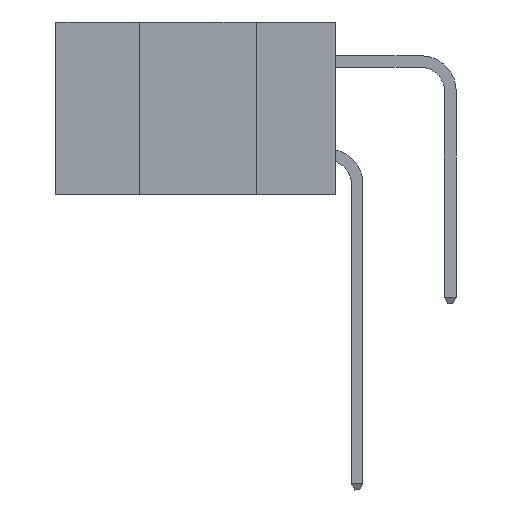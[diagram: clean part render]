
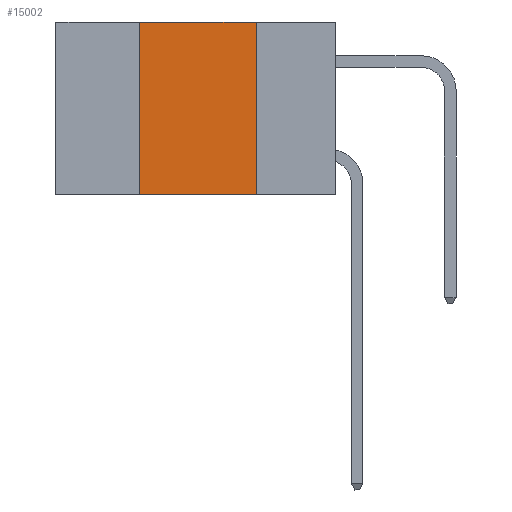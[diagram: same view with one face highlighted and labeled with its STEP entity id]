
A CAD part, left-side view. The second image highlights one B-rep face of the part: STEP entity #15002.
In plain terms, the highlighted planar face has unit normal (-1, 0, 0).
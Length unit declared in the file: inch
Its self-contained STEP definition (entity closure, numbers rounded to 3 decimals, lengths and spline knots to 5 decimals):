
#491 = CARTESIAN_POINT ( 'NONE',  ( 0., 0.17, 0. ) ) ;
#809 = LINE ( 'NONE', #27666, #2516 ) ;
#2391 = ORIENTED_EDGE ( 'NONE', *, *, #9211, .F. ) ;
#2492 = AXIS2_PLACEMENT_3D ( 'NONE', #27152, #17846, #4765 ) ;
#2516 = VECTOR ( 'NONE', #16342, 39.37008 ) ;
#4765 = DIRECTION ( 'NONE',  ( 0., 0., -1. ) ) ;
#4841 = DIRECTION ( 'NONE',  ( 0., 0., 1. ) ) ;
#5401 = LINE ( 'NONE', #14250, #13706 ) ;
#5570 = VERTEX_POINT ( 'NONE', #27965 ) ;
#7860 = CARTESIAN_POINT ( 'NONE',  ( 0., 0.17, 0. ) ) ;
#8285 = DIRECTION ( 'NONE',  ( 0., 0., -1. ) ) ;
#9211 = EDGE_CURVE ( 'NONE', #12813, #18475, #12354, .T. ) ;
#9977 = EDGE_CURVE ( 'NONE', #17232, #18475, #809, .T. ) ;
#11449 = ORIENTED_EDGE ( 'NONE', *, *, #23088, .F. ) ;
#12354 = LINE ( 'NONE', #7860, #24867 ) ;
#12586 = EDGE_LOOP ( 'NONE', ( #2391, #12917, #11449, #15328 ) ) ;
#12813 = VERTEX_POINT ( 'NONE', #491 ) ;
#12845 = CARTESIAN_POINT ( 'NONE',  ( 0., 0.6, 0. ) ) ;
#12917 = ORIENTED_EDGE ( 'NONE', *, *, #27678, .F. ) ;
#13706 = VECTOR ( 'NONE', #4841, 39.37008 ) ;
#14250 = CARTESIAN_POINT ( 'NONE',  ( 0., 0.42, 0. ) ) ;
#14514 = CARTESIAN_POINT ( 'NONE',  ( 0., 0.17, -0.37 ) ) ;
#14952 = VECTOR ( 'NONE', #22011, 39.37008 ) ;
#15002 = ADVANCED_FACE ( 'NONE', ( #15665 ), #22932, .F. ) ;
#15328 = ORIENTED_EDGE ( 'NONE', *, *, #9977, .T. ) ;
#15665 = FACE_OUTER_BOUND ( 'NONE', #12586, .T. ) ;
#16342 = DIRECTION ( 'NONE',  ( 0., -1., 0. ) ) ;
#17232 = VERTEX_POINT ( 'NONE', #17411 ) ;
#17411 = CARTESIAN_POINT ( 'NONE',  ( 0., 0.42, -0.37 ) ) ;
#17846 = DIRECTION ( 'NONE',  ( 1., 0., 0. ) ) ;
#18475 = VERTEX_POINT ( 'NONE', #14514 ) ;
#22011 = DIRECTION ( 'NONE',  ( 0., -1., 0. ) ) ;
#22932 = PLANE ( 'NONE',  #2492 ) ;
#23088 = EDGE_CURVE ( 'NONE', #17232, #5570, #5401, .T. ) ;
#24867 = VECTOR ( 'NONE', #8285, 39.37008 ) ;
#26505 = LINE ( 'NONE', #12845, #14952 ) ;
#27152 = CARTESIAN_POINT ( 'NONE',  ( 0., 0.6, 0. ) ) ;
#27666 = CARTESIAN_POINT ( 'NONE',  ( 0., 0.6, -0.37 ) ) ;
#27678 = EDGE_CURVE ( 'NONE', #5570, #12813, #26505, .T. ) ;
#27965 = CARTESIAN_POINT ( 'NONE',  ( 0., 0.42, 0. ) ) ;
